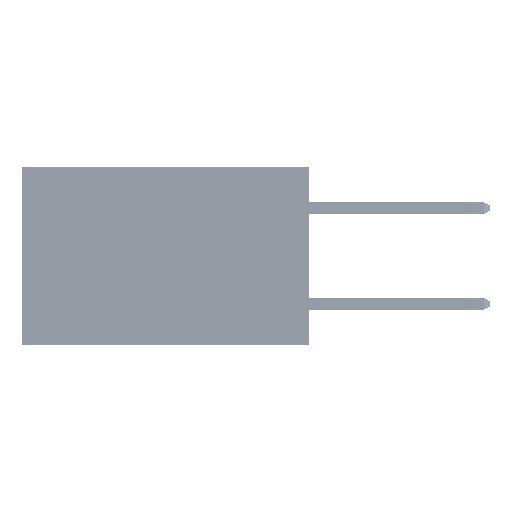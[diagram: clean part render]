
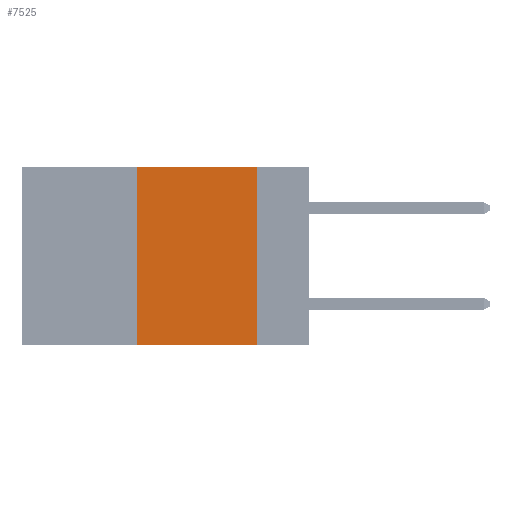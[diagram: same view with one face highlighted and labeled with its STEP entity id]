
A CAD part, left-side view. The second image highlights one B-rep face of the part: STEP entity #7525.
In plain terms, the highlighted planar face has unit normal (-1, 0, 0).
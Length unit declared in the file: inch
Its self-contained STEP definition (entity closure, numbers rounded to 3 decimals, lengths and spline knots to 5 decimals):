
#879 = LINE ( 'NONE', #26048, #45640 ) ;
#3293 = VERTEX_POINT ( 'NONE', #42891 ) ;
#6541 = EDGE_CURVE ( 'NONE', #43078, #25718, #20028, .T. ) ;
#7525 = ADVANCED_FACE ( 'NONE', ( #15711 ), #18963, .F. ) ;
#7564 = DIRECTION ( 'NONE',  ( 0., -1., 0. ) ) ;
#7816 = EDGE_LOOP ( 'NONE', ( #14968, #36415, #44368, #32407 ) ) ;
#9831 = LINE ( 'NONE', #10263, #24157 ) ;
#10263 = CARTESIAN_POINT ( 'NONE',  ( 0., 0.11, 0. ) ) ;
#13385 = EDGE_CURVE ( 'NONE', #25718, #21442, #9831, .T. ) ;
#14759 = DIRECTION ( 'NONE',  ( 0., 0., -1. ) ) ;
#14968 = ORIENTED_EDGE ( 'NONE', *, *, #13385, .F. ) ;
#15711 = FACE_OUTER_BOUND ( 'NONE', #7816, .T. ) ;
#15737 = CARTESIAN_POINT ( 'NONE',  ( 0., 0.11, 0. ) ) ;
#18963 = PLANE ( 'NONE',  #31543 ) ;
#20028 = LINE ( 'NONE', #35067, #37932 ) ;
#21442 = VERTEX_POINT ( 'NONE', #47160 ) ;
#22463 = EDGE_CURVE ( 'NONE', #3293, #21442, #35205, .T. ) ;
#22717 = DIRECTION ( 'NONE',  ( 0., 0., 1. ) ) ;
#24157 = VECTOR ( 'NONE', #14759, 39.37008 ) ;
#25075 = VECTOR ( 'NONE', #7564, 39.37008 ) ;
#25718 = VERTEX_POINT ( 'NONE', #15737 ) ;
#26048 = CARTESIAN_POINT ( 'NONE',  ( 0., 0.36, 0. ) ) ;
#29996 = DIRECTION ( 'NONE',  ( 0., 0., -1. ) ) ;
#31543 = AXIS2_PLACEMENT_3D ( 'NONE', #45636, #33831, #29996 ) ;
#32407 = ORIENTED_EDGE ( 'NONE', *, *, #22463, .T. ) ;
#33831 = DIRECTION ( 'NONE',  ( 1., 0., 0. ) ) ;
#35067 = CARTESIAN_POINT ( 'NONE',  ( 0., 0.6, 0. ) ) ;
#35205 = LINE ( 'NONE', #45918, #25075 ) ;
#35748 = CARTESIAN_POINT ( 'NONE',  ( 0., 0.36, 0. ) ) ;
#36415 = ORIENTED_EDGE ( 'NONE', *, *, #6541, .F. ) ;
#37891 = EDGE_CURVE ( 'NONE', #3293, #43078, #879, .T. ) ;
#37932 = VECTOR ( 'NONE', #46868, 39.37008 ) ;
#42891 = CARTESIAN_POINT ( 'NONE',  ( 0., 0.36, -0.37 ) ) ;
#43078 = VERTEX_POINT ( 'NONE', #35748 ) ;
#44368 = ORIENTED_EDGE ( 'NONE', *, *, #37891, .F. ) ;
#45636 = CARTESIAN_POINT ( 'NONE',  ( 0., 0.6, 0. ) ) ;
#45640 = VECTOR ( 'NONE', #22717, 39.37008 ) ;
#45918 = CARTESIAN_POINT ( 'NONE',  ( 0., 0.6, -0.37 ) ) ;
#46868 = DIRECTION ( 'NONE',  ( 0., -1., 0. ) ) ;
#47160 = CARTESIAN_POINT ( 'NONE',  ( 0., 0.11, -0.37 ) ) ;
